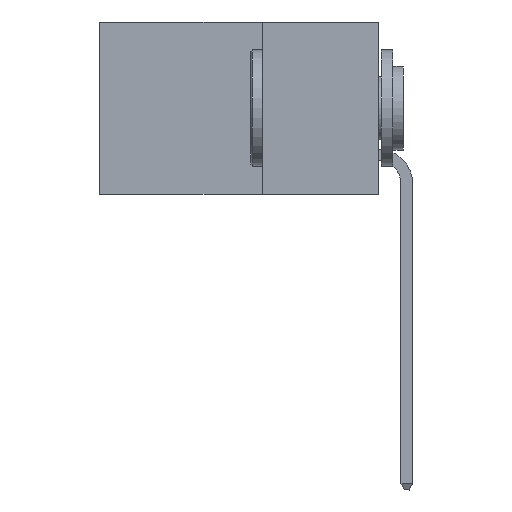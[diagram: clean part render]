
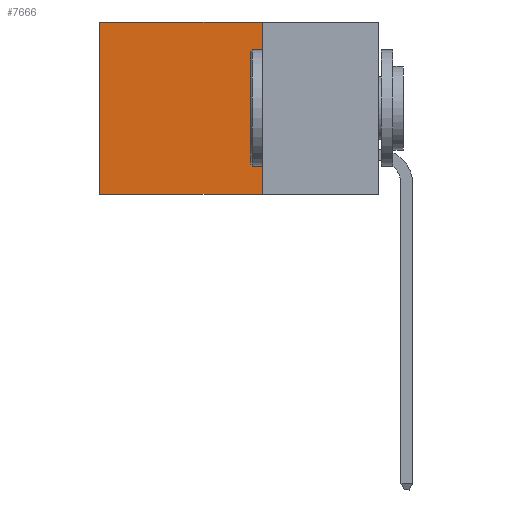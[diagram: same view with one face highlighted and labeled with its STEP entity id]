
A CAD part, left-side view. The second image highlights one B-rep face of the part: STEP entity #7666.
In plain terms, the highlighted planar face has unit normal (-1, 0, 0).
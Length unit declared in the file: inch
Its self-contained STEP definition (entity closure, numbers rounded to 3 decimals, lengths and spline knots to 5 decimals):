
#1486 = VECTOR ( 'NONE', #8387, 39.37008 ) ;
#1739 = VERTEX_POINT ( 'NONE', #4491 ) ;
#3924 = LINE ( 'NONE', #8533, #1486 ) ;
#4102 = FACE_OUTER_BOUND ( 'NONE', #13042, .T. ) ;
#4438 = CARTESIAN_POINT ( 'NONE',  ( 0.2615, 0.6, 0. ) ) ;
#4466 = CARTESIAN_POINT ( 'NONE',  ( 0.2615, 0.25, 0. ) ) ;
#4491 = CARTESIAN_POINT ( 'NONE',  ( 0.2615, 0.6, -0.37 ) ) ;
#4929 = EDGE_CURVE ( 'NONE', #13527, #8790, #5684, .T. ) ;
#4944 = VECTOR ( 'NONE', #10111, 39.37008 ) ;
#5317 = DIRECTION ( 'NONE',  ( 0., 0., -1. ) ) ;
#5499 = ORIENTED_EDGE ( 'NONE', *, *, #13728, .F. ) ;
#5512 = LINE ( 'NONE', #12912, #7253 ) ;
#5684 = LINE ( 'NONE', #11266, #4944 ) ;
#6266 = LINE ( 'NONE', #11987, #10039 ) ;
#6279 = DIRECTION ( 'NONE',  ( 0., 0., -1. ) ) ;
#6691 = CARTESIAN_POINT ( 'NONE',  ( 0.2615, 0.25, -0.37 ) ) ;
#7253 = VECTOR ( 'NONE', #5317, 39.37008 ) ;
#7466 = ORIENTED_EDGE ( 'NONE', *, *, #4929, .T. ) ;
#7666 = ADVANCED_FACE ( 'NONE', ( #4102 ), #9759, .F. ) ;
#7950 = AXIS2_PLACEMENT_3D ( 'NONE', #11994, #13973, #6279 ) ;
#8138 = EDGE_CURVE ( 'NONE', #8790, #1739, #5512, .T. ) ;
#8206 = EDGE_CURVE ( 'NONE', #10097, #1739, #6266, .T. ) ;
#8387 = DIRECTION ( 'NONE',  ( 0., 0., -1. ) ) ;
#8533 = CARTESIAN_POINT ( 'NONE',  ( 0.2615, 0.25, -0.37 ) ) ;
#8790 = VERTEX_POINT ( 'NONE', #4438 ) ;
#9669 = ORIENTED_EDGE ( 'NONE', *, *, #8138, .T. ) ;
#9759 = PLANE ( 'NONE',  #7950 ) ;
#10039 = VECTOR ( 'NONE', #14033, 39.37008 ) ;
#10097 = VERTEX_POINT ( 'NONE', #6691 ) ;
#10111 = DIRECTION ( 'NONE',  ( 0., 1., 0. ) ) ;
#11266 = CARTESIAN_POINT ( 'NONE',  ( 0.2615, 0.25, 0. ) ) ;
#11987 = CARTESIAN_POINT ( 'NONE',  ( 0.2615, 0.25, -0.37 ) ) ;
#11994 = CARTESIAN_POINT ( 'NONE',  ( 0.2615, 0.25, -0.37 ) ) ;
#12912 = CARTESIAN_POINT ( 'NONE',  ( 0.2615, 0.6, -0.37 ) ) ;
#13042 = EDGE_LOOP ( 'NONE', ( #9669, #13841, #5499, #7466 ) ) ;
#13527 = VERTEX_POINT ( 'NONE', #4466 ) ;
#13728 = EDGE_CURVE ( 'NONE', #13527, #10097, #3924, .T. ) ;
#13841 = ORIENTED_EDGE ( 'NONE', *, *, #8206, .F. ) ;
#13973 = DIRECTION ( 'NONE',  ( 1., 0., 0. ) ) ;
#14033 = DIRECTION ( 'NONE',  ( 0., 1., 0. ) ) ;
